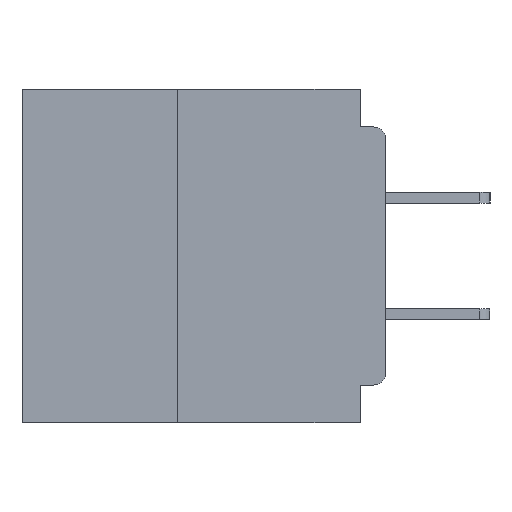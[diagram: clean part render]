
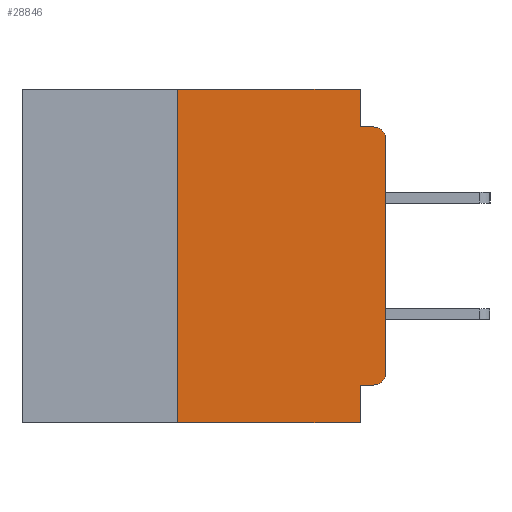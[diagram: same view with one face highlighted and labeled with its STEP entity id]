
A CAD part, left-side view. The second image highlights one B-rep face of the part: STEP entity #28846.
In plain terms, the highlighted planar face has unit normal (-1, 0, 0).
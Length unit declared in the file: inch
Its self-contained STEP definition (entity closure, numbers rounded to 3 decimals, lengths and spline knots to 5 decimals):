
#12 = VECTOR ( 'NONE', #33251, 39.37008 ) ;
#572 = CARTESIAN_POINT ( 'NONE',  ( 0., 0.031, -0.045 ) ) ;
#765 = LINE ( 'NONE', #23463, #41494 ) ;
#1008 = ORIENTED_EDGE ( 'NONE', *, *, #47312, .F. ) ;
#1988 = DIRECTION ( 'NONE',  ( 0., -1., 0. ) ) ;
#2043 = ORIENTED_EDGE ( 'NONE', *, *, #37459, .T. ) ;
#4519 = VECTOR ( 'NONE', #1988, 39.37008 ) ;
#4694 = CARTESIAN_POINT ( 'NONE',  ( 0., 0.015, -0.355 ) ) ;
#5512 = ORIENTED_EDGE ( 'NONE', *, *, #37608, .F. ) ;
#6038 = EDGE_CURVE ( 'NONE', #33449, #24113, #43813, .T. ) ;
#7568 = ORIENTED_EDGE ( 'NONE', *, *, #38967, .T. ) ;
#7700 = CARTESIAN_POINT ( 'NONE',  ( 0., 0., -0.355 ) ) ;
#7902 = DIRECTION ( 'NONE',  ( 1., 0., 0. ) ) ;
#10639 = LINE ( 'NONE', #21401, #12 ) ;
#10777 = DIRECTION ( 'NONE',  ( 0., 0., -1. ) ) ;
#10881 = LINE ( 'NONE', #15290, #29383 ) ;
#11063 = EDGE_CURVE ( 'NONE', #17168, #25787, #25587, .T. ) ;
#11844 = AXIS2_PLACEMENT_3D ( 'NONE', #18247, #45651, #22193 ) ;
#12446 = AXIS2_PLACEMENT_3D ( 'NONE', #12738, #40217, #16713 ) ;
#12738 = CARTESIAN_POINT ( 'NONE',  ( 0., 0.015, -0.06 ) ) ;
#13023 = VERTEX_POINT ( 'NONE', #46080 ) ;
#13813 = ORIENTED_EDGE ( 'NONE', *, *, #38822, .F. ) ;
#15290 = CARTESIAN_POINT ( 'NONE',  ( 0., 0.25, -0.4 ) ) ;
#15685 = CARTESIAN_POINT ( 'NONE',  ( 0., 0., 0. ) ) ;
#16561 = ORIENTED_EDGE ( 'NONE', *, *, #11063, .T. ) ;
#16713 = DIRECTION ( 'NONE',  ( 0., 0., -1. ) ) ;
#16937 = EDGE_CURVE ( 'NONE', #45916, #37993, #41063, .T. ) ;
#17168 = VERTEX_POINT ( 'NONE', #19712 ) ;
#18247 = CARTESIAN_POINT ( 'NONE',  ( 0., 0.015, -0.34 ) ) ;
#18306 = VERTEX_POINT ( 'NONE', #46507 ) ;
#18627 = DIRECTION ( 'NONE',  ( 0., 0., -1. ) ) ;
#18960 = CARTESIAN_POINT ( 'NONE',  ( 0., 0., -0.34 ) ) ;
#19712 = CARTESIAN_POINT ( 'NONE',  ( 0., 0.25, -0.4 ) ) ;
#19844 = EDGE_CURVE ( 'NONE', #37993, #18306, #10639, .T. ) ;
#20763 = EDGE_LOOP ( 'NONE', ( #7568, #41264, #49165, #29791, #1008, #5512, #16561, #13813, #45855, #2043 ) ) ;
#21401 = CARTESIAN_POINT ( 'NONE',  ( 0., 0., -0.045 ) ) ;
#22193 = DIRECTION ( 'NONE',  ( 0., 0., -1. ) ) ;
#23463 = CARTESIAN_POINT ( 'NONE',  ( 0., 0.437, 0. ) ) ;
#23683 = VECTOR ( 'NONE', #18627, 39.37008 ) ;
#23770 = DIRECTION ( 'NONE',  ( 0., 0., -1. ) ) ;
#24113 = VERTEX_POINT ( 'NONE', #27011 ) ;
#24129 = FACE_OUTER_BOUND ( 'NONE', #20763, .T. ) ;
#25587 = LINE ( 'NONE', #33602, #4519 ) ;
#25787 = VERTEX_POINT ( 'NONE', #35068 ) ;
#25962 = EDGE_CURVE ( 'NONE', #13023, #18306, #26304, .T. ) ;
#26304 = CIRCLE ( 'NONE', #12446, 0.015 ) ;
#26769 = LINE ( 'NONE', #15685, #28004 ) ;
#27011 = CARTESIAN_POINT ( 'NONE',  ( 0., 0.031, -0.355 ) ) ;
#28004 = VECTOR ( 'NONE', #31505, 39.37008 ) ;
#28846 = ADVANCED_FACE ( 'NONE', ( #24129 ), #47220, .F. ) ;
#29383 = VECTOR ( 'NONE', #31119, 39.37008 ) ;
#29791 = ORIENTED_EDGE ( 'NONE', *, *, #16937, .F. ) ;
#31041 = CARTESIAN_POINT ( 'NONE',  ( 0., 0.25, 0. ) ) ;
#31119 = DIRECTION ( 'NONE',  ( 0., 0., 1. ) ) ;
#31298 = DIRECTION ( 'NONE',  ( 0., 1., 0. ) ) ;
#31505 = DIRECTION ( 'NONE',  ( 0., 0., 1. ) ) ;
#32542 = VERTEX_POINT ( 'NONE', #31041 ) ;
#33251 = DIRECTION ( 'NONE',  ( 0., -1., 0. ) ) ;
#33449 = VERTEX_POINT ( 'NONE', #4694 ) ;
#33602 = CARTESIAN_POINT ( 'NONE',  ( 0., 0.437, -0.4 ) ) ;
#34313 = CARTESIAN_POINT ( 'NONE',  ( 0., 0.031, 0. ) ) ;
#34406 = CARTESIAN_POINT ( 'NONE',  ( 0., 0.031, -0.4 ) ) ;
#34910 = VERTEX_POINT ( 'NONE', #18960 ) ;
#35068 = CARTESIAN_POINT ( 'NONE',  ( 0., 0.031, -0.4 ) ) ;
#36855 = AXIS2_PLACEMENT_3D ( 'NONE', #43302, #7902, #23770 ) ;
#37459 = EDGE_CURVE ( 'NONE', #33449, #34910, #47118, .T. ) ;
#37608 = EDGE_CURVE ( 'NONE', #17168, #32542, #10881, .T. ) ;
#37993 = VERTEX_POINT ( 'NONE', #572 ) ;
#38822 = EDGE_CURVE ( 'NONE', #24113, #25787, #44532, .T. ) ;
#38967 = EDGE_CURVE ( 'NONE', #34910, #13023, #26769, .T. ) ;
#40217 = DIRECTION ( 'NONE',  ( -1., 0., 0. ) ) ;
#41063 = LINE ( 'NONE', #34313, #42273 ) ;
#41264 = ORIENTED_EDGE ( 'NONE', *, *, #25962, .T. ) ;
#41494 = VECTOR ( 'NONE', #46914, 39.37008 ) ;
#42273 = VECTOR ( 'NONE', #10777, 39.37008 ) ;
#42575 = VECTOR ( 'NONE', #31298, 39.37008 ) ;
#43302 = CARTESIAN_POINT ( 'NONE',  ( 0., 0.437, 0. ) ) ;
#43813 = LINE ( 'NONE', #7700, #42575 ) ;
#44532 = LINE ( 'NONE', #34406, #23683 ) ;
#45651 = DIRECTION ( 'NONE',  ( -1., 0., 0. ) ) ;
#45855 = ORIENTED_EDGE ( 'NONE', *, *, #6038, .F. ) ;
#45916 = VERTEX_POINT ( 'NONE', #46190 ) ;
#46080 = CARTESIAN_POINT ( 'NONE',  ( 0., 0., -0.06 ) ) ;
#46190 = CARTESIAN_POINT ( 'NONE',  ( 0., 0.031, 0. ) ) ;
#46507 = CARTESIAN_POINT ( 'NONE',  ( 0., 0.015, -0.045 ) ) ;
#46914 = DIRECTION ( 'NONE',  ( 0., -1., 0. ) ) ;
#47118 = CIRCLE ( 'NONE', #11844, 0.015 ) ;
#47220 = PLANE ( 'NONE',  #36855 ) ;
#47312 = EDGE_CURVE ( 'NONE', #32542, #45916, #765, .T. ) ;
#49165 = ORIENTED_EDGE ( 'NONE', *, *, #19844, .F. ) ;
